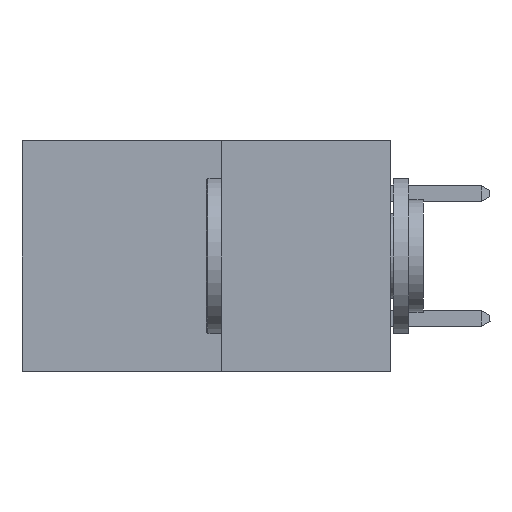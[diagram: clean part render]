
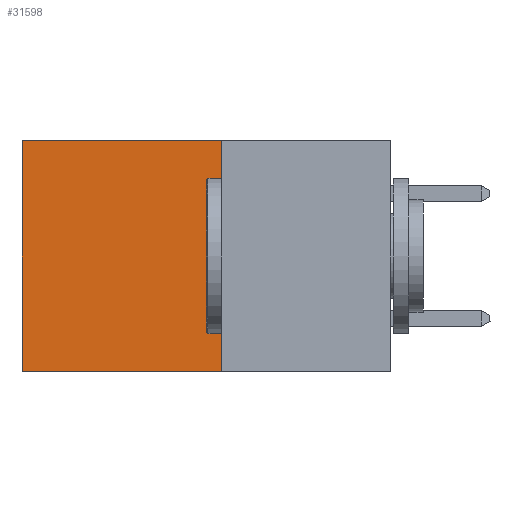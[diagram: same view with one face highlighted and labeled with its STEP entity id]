
A CAD part, left-side view. The second image highlights one B-rep face of the part: STEP entity #31598.
In plain terms, the highlighted planar face has unit normal (-1, 0, 0).
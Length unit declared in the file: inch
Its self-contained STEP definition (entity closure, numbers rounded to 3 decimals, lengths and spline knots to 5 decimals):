
#529 = CARTESIAN_POINT ( 'NONE',  ( 0.277, 0.59, -0.37 ) ) ;
#663 = CARTESIAN_POINT ( 'NONE',  ( 0.277, 0.27, -0.37 ) ) ;
#679 = DIRECTION ( 'NONE',  ( 0., 0., -1. ) ) ;
#754 = VECTOR ( 'NONE', #15978, 39.37008 ) ;
#1272 = VERTEX_POINT ( 'NONE', #24704 ) ;
#1999 = EDGE_CURVE ( 'NONE', #1272, #30221, #25806, .T. ) ;
#2580 = LINE ( 'NONE', #12914, #3412 ) ;
#3003 = CARTESIAN_POINT ( 'NONE',  ( 0.277, 0.27, -0.37 ) ) ;
#3279 = DIRECTION ( 'NONE',  ( 0., 1., 0. ) ) ;
#3412 = VECTOR ( 'NONE', #15366, 39.37008 ) ;
#5348 = ORIENTED_EDGE ( 'NONE', *, *, #27139, .F. ) ;
#7389 = DIRECTION ( 'NONE',  ( 0., 1., 0. ) ) ;
#7390 = EDGE_CURVE ( 'NONE', #30961, #1272, #11704, .T. ) ;
#7549 = CARTESIAN_POINT ( 'NONE',  ( 0.277, 0.27, 0. ) ) ;
#8450 = ORIENTED_EDGE ( 'NONE', *, *, #7390, .T. ) ;
#11704 = LINE ( 'NONE', #7549, #30568 ) ;
#12091 = LINE ( 'NONE', #663, #24147 ) ;
#12914 = CARTESIAN_POINT ( 'NONE',  ( 0.277, 0.27, -0.37 ) ) ;
#13492 = PLANE ( 'NONE',  #27500 ) ;
#14918 = VERTEX_POINT ( 'NONE', #3003 ) ;
#15366 = DIRECTION ( 'NONE',  ( 0., 0., -1. ) ) ;
#15978 = DIRECTION ( 'NONE',  ( 0., 0., -1. ) ) ;
#16008 = CARTESIAN_POINT ( 'NONE',  ( 0.277, 0.59, -0.37 ) ) ;
#16049 = DIRECTION ( 'NONE',  ( 1., 0., 0. ) ) ;
#19821 = EDGE_CURVE ( 'NONE', #14918, #30221, #12091, .T. ) ;
#21410 = EDGE_LOOP ( 'NONE', ( #27752, #27932, #5348, #8450 ) ) ;
#23220 = FACE_OUTER_BOUND ( 'NONE', #21410, .T. ) ;
#24147 = VECTOR ( 'NONE', #3279, 39.37008 ) ;
#24704 = CARTESIAN_POINT ( 'NONE',  ( 0.277, 0.59, 0. ) ) ;
#25806 = LINE ( 'NONE', #16008, #754 ) ;
#27139 = EDGE_CURVE ( 'NONE', #30961, #14918, #2580, .T. ) ;
#27500 = AXIS2_PLACEMENT_3D ( 'NONE', #31419, #16049, #679 ) ;
#27752 = ORIENTED_EDGE ( 'NONE', *, *, #1999, .T. ) ;
#27932 = ORIENTED_EDGE ( 'NONE', *, *, #19821, .F. ) ;
#29022 = CARTESIAN_POINT ( 'NONE',  ( 0.277, 0.27, 0. ) ) ;
#30221 = VERTEX_POINT ( 'NONE', #529 ) ;
#30568 = VECTOR ( 'NONE', #7389, 39.37008 ) ;
#30961 = VERTEX_POINT ( 'NONE', #29022 ) ;
#31419 = CARTESIAN_POINT ( 'NONE',  ( 0.277, 0.27, -0.37 ) ) ;
#31598 = ADVANCED_FACE ( 'NONE', ( #23220 ), #13492, .F. ) ;
